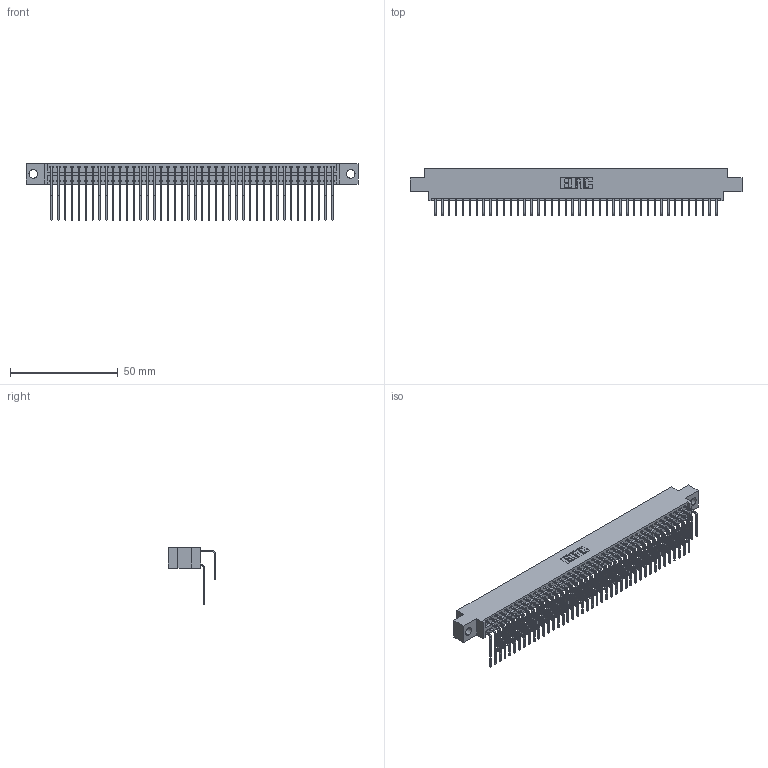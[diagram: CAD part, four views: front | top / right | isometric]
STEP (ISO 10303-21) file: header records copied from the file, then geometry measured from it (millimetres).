
FILE_DESCRIPTION (( 'STEP AP203' ), '1' );
FILE_NAME ('346-084-558-804.STEP', '2022-05-25T20:55:21', ( '' ), ( '' ), 'SwSTEP 2.0', 'SolidWorks 2020', '' );
FILE_SCHEMA (( 'CONFIG_CONTROL_DESIGN' ));
Length unit declared in the file: inch
Products named in the file (4): 345-292-001_558 Tail - 2; 346-084-558-804; 345-292-001_558 559 Tail - 1; 346 Part_0.170 Offset - 0.156 Dia-TH
Assembly tree (85 placements, depth 2):
  346-084-558-804
    346 Part_0.170 Offset - 0.156 Dia-TH
    345-292-001_558 559 Tail - 1  x42
    345-292-001_558 Tail - 2  x42
Bounding box: 153.92 x 22.16 x 26.16 mm (x, y, z)
Volume: 15233.5 mm3; surface area: 23291.7 mm2
Topology: 85 solids, 85 shells, 4676 faces, 13901 edges, 9154 vertices
Faces by surface type: plane 3202, cylinder 1474
Entity records: 29745 total; most frequent: CARTESIAN_POINT 4961, ORIENTED_EDGE 4842, DIRECTION 4393, EDGE_CURVE 2421, VECTOR 2081, LINE 2081, VERTEX_POINT 1610, AXIS2_PLACEMENT_3D 1156
